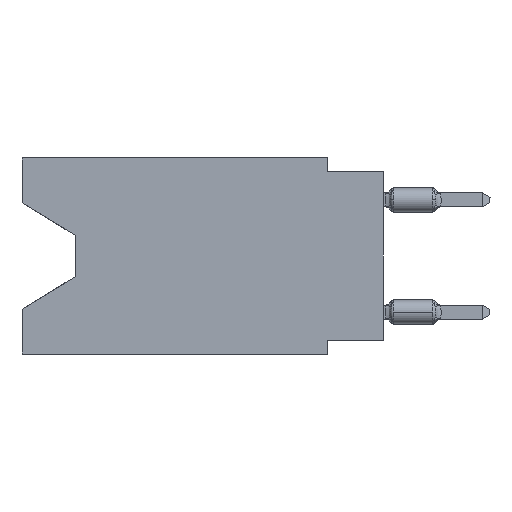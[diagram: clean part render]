
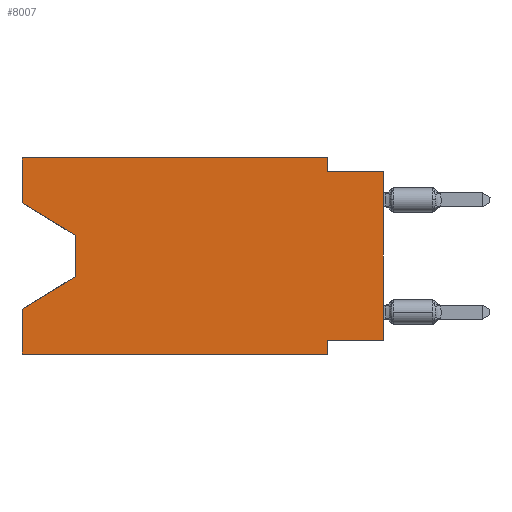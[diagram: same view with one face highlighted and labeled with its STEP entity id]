
A CAD part, left-side view. The second image highlights one B-rep face of the part: STEP entity #8007.
In plain terms, the highlighted planar face has unit normal (-1, 0, 0).
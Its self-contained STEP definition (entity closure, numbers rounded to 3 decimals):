
#81 = VECTOR ( 'NONE', #12853, 1000. ) ;
#218 = ORIENTED_EDGE ( 'NONE', *, *, #5499, .F. ) ;
#311 = LINE ( 'NONE', #20885, #2287 ) ;
#465 = PLANE ( 'NONE',  #16840 ) ;
#660 = CARTESIAN_POINT ( 'NONE',  ( 0., 16.383, 0. ) ) ;
#670 = EDGE_CURVE ( 'NONE', #19553, #23008, #14706, .T. ) ;
#696 = CARTESIAN_POINT ( 'NONE',  ( 0., 0., -0.635 ) ) ;
#734 = DIRECTION ( 'NONE',  ( 0., 0.855, -0.519 ) ) ;
#1103 = CARTESIAN_POINT ( 'NONE',  ( 0., 16.383, -8.89 ) ) ;
#1628 = EDGE_CURVE ( 'NONE', #13485, #6874, #1664, .T. ) ;
#1664 = LINE ( 'NONE', #14720, #14282 ) ;
#2287 = VECTOR ( 'NONE', #3635, 1000. ) ;
#2765 = EDGE_CURVE ( 'NONE', #11342, #14040, #23190, .T. ) ;
#3633 = VECTOR ( 'NONE', #20991, 1000. ) ;
#3635 = DIRECTION ( 'NONE',  ( 0., 0., 1. ) ) ;
#3721 = CARTESIAN_POINT ( 'NONE',  ( 0., 16.383, -6.852 ) ) ;
#4119 = CARTESIAN_POINT ( 'NONE',  ( 0., 0., -0.635 ) ) ;
#4149 = CARTESIAN_POINT ( 'NONE',  ( 0., 16.383, 0. ) ) ;
#4429 = CARTESIAN_POINT ( 'NONE',  ( 0., 13.97, -5.385 ) ) ;
#4490 = CARTESIAN_POINT ( 'NONE',  ( 0., 16.383, 0. ) ) ;
#4533 = EDGE_LOOP ( 'NONE', ( #16059, #6847, #14736, #218, #9901, #14812, #14778, #9814, #12386, #8355, #23883, #5091 ) ) ;
#5091 = ORIENTED_EDGE ( 'NONE', *, *, #7317, .F. ) ;
#5271 = EDGE_CURVE ( 'NONE', #15544, #13485, #6253, .T. ) ;
#5338 = CARTESIAN_POINT ( 'NONE',  ( 0., 2.54, -8.89 ) ) ;
#5499 = EDGE_CURVE ( 'NONE', #13355, #20252, #311, .T. ) ;
#5578 = CARTESIAN_POINT ( 'NONE',  ( 0., 13.97, -3.505 ) ) ;
#5780 = CARTESIAN_POINT ( 'NONE',  ( 0., 0., -8.255 ) ) ;
#6253 = LINE ( 'NONE', #15603, #14470 ) ;
#6847 = ORIENTED_EDGE ( 'NONE', *, *, #1628, .T. ) ;
#6874 = VERTEX_POINT ( 'NONE', #15845 ) ;
#7317 = EDGE_CURVE ( 'NONE', #15544, #18721, #16182, .T. ) ;
#7644 = LINE ( 'NONE', #5780, #15073 ) ;
#8007 = ADVANCED_FACE ( 'NONE', ( #8219 ), #465, .F. ) ;
#8102 = CARTESIAN_POINT ( 'NONE',  ( 0., 2.54, -8.89 ) ) ;
#8219 = FACE_OUTER_BOUND ( 'NONE', #4533, .T. ) ;
#8269 = EDGE_CURVE ( 'NONE', #18721, #18763, #20278, .T. ) ;
#8355 = ORIENTED_EDGE ( 'NONE', *, *, #12569, .F. ) ;
#8473 = EDGE_CURVE ( 'NONE', #18712, #14040, #21002, .T. ) ;
#9667 = DIRECTION ( 'NONE',  ( 0., -1., 0. ) ) ;
#9814 = ORIENTED_EDGE ( 'NONE', *, *, #2765, .T. ) ;
#9901 = ORIENTED_EDGE ( 'NONE', *, *, #11451, .T. ) ;
#10837 = DIRECTION ( 'NONE',  ( 0., -1., 0. ) ) ;
#11034 = CARTESIAN_POINT ( 'NONE',  ( 0., 16.383, 0. ) ) ;
#11342 = VERTEX_POINT ( 'NONE', #17617 ) ;
#11451 = EDGE_CURVE ( 'NONE', #13355, #23008, #12562, .T. ) ;
#11704 = CARTESIAN_POINT ( 'NONE',  ( 0., 2.54, -8.255 ) ) ;
#12007 = DIRECTION ( 'NONE',  ( 0., 0., 1. ) ) ;
#12386 = ORIENTED_EDGE ( 'NONE', *, *, #8473, .F. ) ;
#12562 = LINE ( 'NONE', #1103, #16165 ) ;
#12569 = EDGE_CURVE ( 'NONE', #18763, #18712, #23391, .T. ) ;
#12714 = VECTOR ( 'NONE', #734, 1000. ) ;
#12853 = DIRECTION ( 'NONE',  ( 0., 0., -1. ) ) ;
#13355 = VERTEX_POINT ( 'NONE', #23937 ) ;
#13485 = VERTEX_POINT ( 'NONE', #5578 ) ;
#13962 = CARTESIAN_POINT ( 'NONE',  ( 0., 2.54, -0.635 ) ) ;
#14040 = VERTEX_POINT ( 'NONE', #696 ) ;
#14282 = VECTOR ( 'NONE', #16208, 1000. ) ;
#14470 = VECTOR ( 'NONE', #23224, 1000. ) ;
#14706 = LINE ( 'NONE', #5338, #81 ) ;
#14720 = CARTESIAN_POINT ( 'NONE',  ( 0., 13.97, -3.505 ) ) ;
#14736 = ORIENTED_EDGE ( 'NONE', *, *, #20896, .T. ) ;
#14778 = ORIENTED_EDGE ( 'NONE', *, *, #21491, .F. ) ;
#14812 = ORIENTED_EDGE ( 'NONE', *, *, #670, .F. ) ;
#15073 = VECTOR ( 'NONE', #17123, 1000. ) ;
#15491 = DIRECTION ( 'NONE',  ( 1., 0., 0. ) ) ;
#15544 = VERTEX_POINT ( 'NONE', #22481 ) ;
#15603 = CARTESIAN_POINT ( 'NONE',  ( 0., 16.383, -2.038 ) ) ;
#15845 = CARTESIAN_POINT ( 'NONE',  ( 0., 13.97, -5.385 ) ) ;
#16059 = ORIENTED_EDGE ( 'NONE', *, *, #5271, .T. ) ;
#16165 = VECTOR ( 'NONE', #10837, 1000. ) ;
#16182 = LINE ( 'NONE', #4490, #23225 ) ;
#16208 = DIRECTION ( 'NONE',  ( 0., 0., -1. ) ) ;
#16697 = DIRECTION ( 'NONE',  ( 0., -1., 0. ) ) ;
#16840 = AXIS2_PLACEMENT_3D ( 'NONE', #4149, #15491, #21266 ) ;
#17123 = DIRECTION ( 'NONE',  ( 0., 1., 0. ) ) ;
#17168 = CARTESIAN_POINT ( 'NONE',  ( 0., 0., 0. ) ) ;
#17225 = VECTOR ( 'NONE', #19358, 1000. ) ;
#17617 = CARTESIAN_POINT ( 'NONE',  ( 0., 0., -8.255 ) ) ;
#18712 = VERTEX_POINT ( 'NONE', #13962 ) ;
#18721 = VERTEX_POINT ( 'NONE', #660 ) ;
#18763 = VERTEX_POINT ( 'NONE', #19512 ) ;
#19358 = DIRECTION ( 'NONE',  ( 0., 0., -1. ) ) ;
#19512 = CARTESIAN_POINT ( 'NONE',  ( 0., 2.54, 0. ) ) ;
#19553 = VERTEX_POINT ( 'NONE', #11704 ) ;
#19720 = CARTESIAN_POINT ( 'NONE',  ( 0., 2.54, 0. ) ) ;
#20252 = VERTEX_POINT ( 'NONE', #3721 ) ;
#20278 = LINE ( 'NONE', #11034, #20404 ) ;
#20404 = VECTOR ( 'NONE', #16697, 1000. ) ;
#20885 = CARTESIAN_POINT ( 'NONE',  ( 0., 16.383, 0. ) ) ;
#20896 = EDGE_CURVE ( 'NONE', #6874, #20252, #21304, .T. ) ;
#20991 = DIRECTION ( 'NONE',  ( 0., 0., 1. ) ) ;
#21002 = LINE ( 'NONE', #4119, #24340 ) ;
#21266 = DIRECTION ( 'NONE',  ( 0., 0., -1. ) ) ;
#21304 = LINE ( 'NONE', #4429, #12714 ) ;
#21491 = EDGE_CURVE ( 'NONE', #11342, #19553, #7644, .T. ) ;
#22481 = CARTESIAN_POINT ( 'NONE',  ( 0., 16.383, -2.038 ) ) ;
#23008 = VERTEX_POINT ( 'NONE', #8102 ) ;
#23190 = LINE ( 'NONE', #17168, #3633 ) ;
#23224 = DIRECTION ( 'NONE',  ( 0., -0.855, -0.519 ) ) ;
#23225 = VECTOR ( 'NONE', #12007, 1000. ) ;
#23391 = LINE ( 'NONE', #19720, #17225 ) ;
#23883 = ORIENTED_EDGE ( 'NONE', *, *, #8269, .F. ) ;
#23937 = CARTESIAN_POINT ( 'NONE',  ( 0., 16.383, -8.89 ) ) ;
#24340 = VECTOR ( 'NONE', #9667, 1000. ) ;
